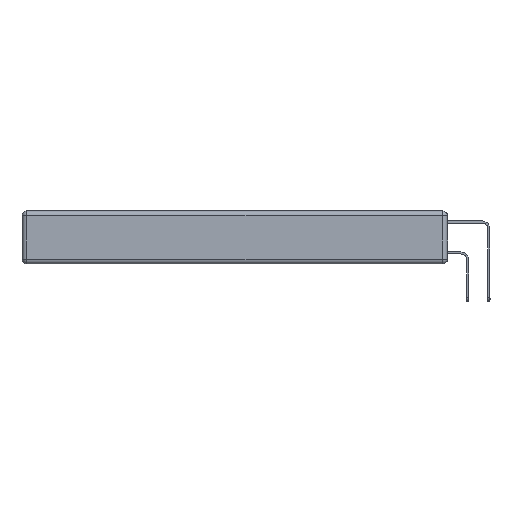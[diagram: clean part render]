
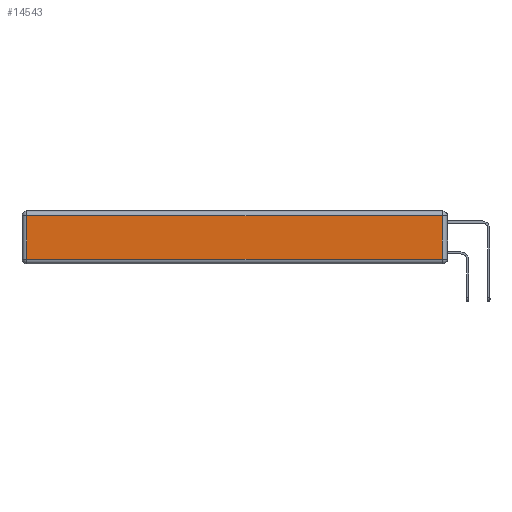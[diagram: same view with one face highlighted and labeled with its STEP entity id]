
A CAD part, left-side view. The second image highlights one B-rep face of the part: STEP entity #14543.
In plain terms, the highlighted planar face has unit normal (-1, 0, 0).
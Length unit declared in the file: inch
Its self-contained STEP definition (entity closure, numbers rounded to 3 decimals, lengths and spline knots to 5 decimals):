
#72 = LINE ( 'NONE', #9651, #1832 ) ;
#297 = ORIENTED_EDGE ( 'NONE', *, *, #8198, .T. ) ;
#543 = CARTESIAN_POINT ( 'NONE',  ( 0., 2.72, -0.313 ) ) ;
#1832 = VECTOR ( 'NONE', #11049, 39.37008 ) ;
#2257 = CARTESIAN_POINT ( 'NONE',  ( 0., 0.03, -0.343 ) ) ;
#3284 = EDGE_LOOP ( 'NONE', ( #10081, #297, #4535, #11169 ) ) ;
#3610 = CARTESIAN_POINT ( 'NONE',  ( 0., 0., -0.343 ) ) ;
#4535 = ORIENTED_EDGE ( 'NONE', *, *, #13206, .T. ) ;
#4553 = EDGE_CURVE ( 'NONE', #12789, #13226, #15254, .T. ) ;
#4724 = CARTESIAN_POINT ( 'NONE',  ( 0., 2.72, -0.343 ) ) ;
#5867 = FACE_OUTER_BOUND ( 'NONE', #3284, .T. ) ;
#6133 = DIRECTION ( 'NONE',  ( 0., 0., -1. ) ) ;
#7403 = VERTEX_POINT ( 'NONE', #11103 ) ;
#7425 = PLANE ( 'NONE',  #15002 ) ;
#8198 = EDGE_CURVE ( 'NONE', #13226, #7403, #15463, .T. ) ;
#8404 = DIRECTION ( 'NONE',  ( 0., 0., 1. ) ) ;
#8531 = CARTESIAN_POINT ( 'NONE',  ( 0., 0.03, -0.313 ) ) ;
#9352 = DIRECTION ( 'NONE',  ( -1., 0., 0. ) ) ;
#9651 = CARTESIAN_POINT ( 'NONE',  ( 0., 2.75, -0.03 ) ) ;
#10081 = ORIENTED_EDGE ( 'NONE', *, *, #4553, .T. ) ;
#10462 = CARTESIAN_POINT ( 'NONE',  ( 0., 0., -0.313 ) ) ;
#11049 = DIRECTION ( 'NONE',  ( 0., 1., 0. ) ) ;
#11103 = CARTESIAN_POINT ( 'NONE',  ( 0., 0.03, -0.03 ) ) ;
#11169 = ORIENTED_EDGE ( 'NONE', *, *, #13655, .T. ) ;
#11453 = VECTOR ( 'NONE', #6133, 39.37008 ) ;
#11784 = DIRECTION ( 'NONE',  ( 0., -1., 0. ) ) ;
#11842 = DIRECTION ( 'NONE',  ( 0., 0., 1. ) ) ;
#12789 = VERTEX_POINT ( 'NONE', #543 ) ;
#13206 = EDGE_CURVE ( 'NONE', #7403, #15229, #72, .T. ) ;
#13226 = VERTEX_POINT ( 'NONE', #8531 ) ;
#13383 = VECTOR ( 'NONE', #11784, 39.37008 ) ;
#13553 = CARTESIAN_POINT ( 'NONE',  ( 0., 2.72, -0.03 ) ) ;
#13556 = VECTOR ( 'NONE', #11842, 39.37008 ) ;
#13655 = EDGE_CURVE ( 'NONE', #15229, #12789, #15515, .T. ) ;
#14543 = ADVANCED_FACE ( 'NONE', ( #5867 ), #7425, .T. ) ;
#15002 = AXIS2_PLACEMENT_3D ( 'NONE', #3610, #9352, #8404 ) ;
#15229 = VERTEX_POINT ( 'NONE', #13553 ) ;
#15254 = LINE ( 'NONE', #10462, #13383 ) ;
#15463 = LINE ( 'NONE', #2257, #13556 ) ;
#15515 = LINE ( 'NONE', #4724, #11453 ) ;
